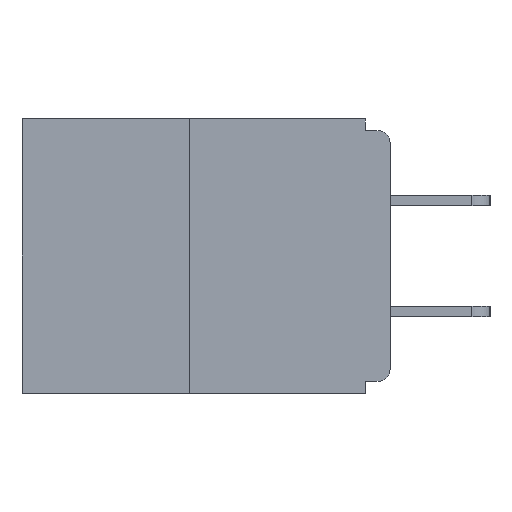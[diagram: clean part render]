
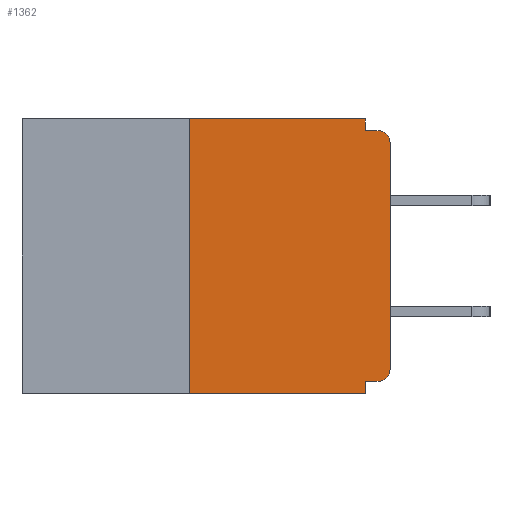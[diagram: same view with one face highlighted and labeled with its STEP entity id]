
A CAD part, left-side view. The second image highlights one B-rep face of the part: STEP entity #1362.
In plain terms, the highlighted planar face has unit normal (-1, 0, 0).
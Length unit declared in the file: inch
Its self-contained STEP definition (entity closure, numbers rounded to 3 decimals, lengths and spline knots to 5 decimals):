
#158 = LINE ( 'NONE', #11465, #11096 ) ;
#204 = DIRECTION ( 'NONE',  ( -1., 0., 0. ) ) ;
#571 = ORIENTED_EDGE ( 'NONE', *, *, #6192, .F. ) ;
#723 = AXIS2_PLACEMENT_3D ( 'NONE', #12080, #2007, #2916 ) ;
#763 = PLANE ( 'NONE',  #6001 ) ;
#1172 = LINE ( 'NONE', #11115, #5064 ) ;
#1209 = CARTESIAN_POINT ( 'NONE',  ( 0., 0.015, -0.313 ) ) ;
#1335 = CARTESIAN_POINT ( 'NONE',  ( 0., 0.25, 0. ) ) ;
#1362 = ADVANCED_FACE ( 'NONE', ( #8601 ), #763, .F. ) ;
#1392 = LINE ( 'NONE', #1335, #8775 ) ;
#1396 = EDGE_CURVE ( 'NONE', #1582, #2213, #1859, .T. ) ;
#1582 = VERTEX_POINT ( 'NONE', #6487 ) ;
#1833 = CARTESIAN_POINT ( 'NONE',  ( 0., 0., 0. ) ) ;
#1859 = LINE ( 'NONE', #5750, #3708 ) ;
#1931 = VECTOR ( 'NONE', #9138, 39.37008 ) ;
#1960 = LINE ( 'NONE', #12014, #11684 ) ;
#2007 = DIRECTION ( 'NONE',  ( -1., 0., 0. ) ) ;
#2177 = DIRECTION ( 'NONE',  ( 0., -1., 0. ) ) ;
#2213 = VERTEX_POINT ( 'NONE', #9863 ) ;
#2240 = VERTEX_POINT ( 'NONE', #11836 ) ;
#2329 = ORIENTED_EDGE ( 'NONE', *, *, #9199, .F. ) ;
#2422 = EDGE_CURVE ( 'NONE', #8087, #2213, #12894, .T. ) ;
#2466 = ORIENTED_EDGE ( 'NONE', *, *, #7427, .F. ) ;
#2494 = VERTEX_POINT ( 'NONE', #4158 ) ;
#2528 = CARTESIAN_POINT ( 'NONE',  ( 0., 0.015, -0.328 ) ) ;
#2592 = ORIENTED_EDGE ( 'NONE', *, *, #1396, .T. ) ;
#2661 = VERTEX_POINT ( 'NONE', #2528 ) ;
#2715 = CIRCLE ( 'NONE', #6135, 0.015 ) ;
#2916 = DIRECTION ( 'NONE',  ( 0., 0., -1. ) ) ;
#3467 = VERTEX_POINT ( 'NONE', #4753 ) ;
#3644 = ORIENTED_EDGE ( 'NONE', *, *, #7300, .T. ) ;
#3673 = DIRECTION ( 'NONE',  ( 0., 0., -1. ) ) ;
#3708 = VECTOR ( 'NONE', #7577, 39.37008 ) ;
#3961 = EDGE_LOOP ( 'NONE', ( #2466, #2329, #2592, #5324, #8359, #8198, #5655, #3644, #4565, #571 ) ) ;
#4158 = CARTESIAN_POINT ( 'NONE',  ( 0., 0., -0.03 ) ) ;
#4565 = ORIENTED_EDGE ( 'NONE', *, *, #8077, .F. ) ;
#4753 = CARTESIAN_POINT ( 'NONE',  ( 0., 0., -0.313 ) ) ;
#4795 = DIRECTION ( 'NONE',  ( 0., 1., 0. ) ) ;
#4956 = DIRECTION ( 'NONE',  ( 0., 0., 1. ) ) ;
#5064 = VECTOR ( 'NONE', #2177, 39.37008 ) ;
#5247 = CARTESIAN_POINT ( 'NONE',  ( 0., 0.031, -0.343 ) ) ;
#5324 = ORIENTED_EDGE ( 'NONE', *, *, #2422, .F. ) ;
#5332 = DIRECTION ( 'NONE',  ( 0., 0., -1. ) ) ;
#5392 = LINE ( 'NONE', #12874, #10449 ) ;
#5416 = DIRECTION ( 'NONE',  ( 0., 0., 1. ) ) ;
#5655 = ORIENTED_EDGE ( 'NONE', *, *, #8929, .T. ) ;
#5750 = CARTESIAN_POINT ( 'NONE',  ( 0., 0.46, -0.343 ) ) ;
#6001 = AXIS2_PLACEMENT_3D ( 'NONE', #11673, #10699, #3673 ) ;
#6135 = AXIS2_PLACEMENT_3D ( 'NONE', #1209, #204, #9180 ) ;
#6192 = EDGE_CURVE ( 'NONE', #2240, #10383, #158, .T. ) ;
#6487 = CARTESIAN_POINT ( 'NONE',  ( 0., 0.25, -0.343 ) ) ;
#6508 = CARTESIAN_POINT ( 'NONE',  ( 0., 0.015, -0.015 ) ) ;
#7300 = EDGE_CURVE ( 'NONE', #2494, #10951, #9175, .T. ) ;
#7427 = EDGE_CURVE ( 'NONE', #9591, #2240, #1172, .T. ) ;
#7447 = CARTESIAN_POINT ( 'NONE',  ( 0., 0.031, -0.015 ) ) ;
#7577 = DIRECTION ( 'NONE',  ( 0., -1., 0. ) ) ;
#8077 = EDGE_CURVE ( 'NONE', #10383, #10951, #1960, .T. ) ;
#8087 = VERTEX_POINT ( 'NONE', #10831 ) ;
#8198 = ORIENTED_EDGE ( 'NONE', *, *, #8713, .T. ) ;
#8247 = CARTESIAN_POINT ( 'NONE',  ( 0., 0.25, 0. ) ) ;
#8359 = ORIENTED_EDGE ( 'NONE', *, *, #11130, .F. ) ;
#8601 = FACE_OUTER_BOUND ( 'NONE', #3961, .T. ) ;
#8713 = EDGE_CURVE ( 'NONE', #2661, #3467, #2715, .T. ) ;
#8775 = VECTOR ( 'NONE', #5416, 39.37008 ) ;
#8929 = EDGE_CURVE ( 'NONE', #3467, #2494, #11355, .T. ) ;
#8990 = DIRECTION ( 'NONE',  ( 0., -1., 0. ) ) ;
#9138 = DIRECTION ( 'NONE',  ( 0., 0., -1. ) ) ;
#9175 = CIRCLE ( 'NONE', #723, 0.015 ) ;
#9180 = DIRECTION ( 'NONE',  ( 0., 0., -1. ) ) ;
#9199 = EDGE_CURVE ( 'NONE', #1582, #9591, #1392, .T. ) ;
#9538 = VECTOR ( 'NONE', #4956, 39.37008 ) ;
#9591 = VERTEX_POINT ( 'NONE', #8247 ) ;
#9863 = CARTESIAN_POINT ( 'NONE',  ( 0., 0.031, -0.343 ) ) ;
#10383 = VERTEX_POINT ( 'NONE', #7447 ) ;
#10449 = VECTOR ( 'NONE', #4795, 39.37008 ) ;
#10699 = DIRECTION ( 'NONE',  ( 1., 0., 0. ) ) ;
#10831 = CARTESIAN_POINT ( 'NONE',  ( 0., 0.031, -0.328 ) ) ;
#10951 = VERTEX_POINT ( 'NONE', #6508 ) ;
#11096 = VECTOR ( 'NONE', #5332, 39.37008 ) ;
#11115 = CARTESIAN_POINT ( 'NONE',  ( 0., 0.46, 0. ) ) ;
#11130 = EDGE_CURVE ( 'NONE', #2661, #8087, #5392, .T. ) ;
#11355 = LINE ( 'NONE', #1833, #9538 ) ;
#11465 = CARTESIAN_POINT ( 'NONE',  ( 0., 0.031, 0. ) ) ;
#11673 = CARTESIAN_POINT ( 'NONE',  ( 0., 0.46, 0. ) ) ;
#11684 = VECTOR ( 'NONE', #8990, 39.37008 ) ;
#11836 = CARTESIAN_POINT ( 'NONE',  ( 0., 0.031, 0. ) ) ;
#12014 = CARTESIAN_POINT ( 'NONE',  ( 0., 0., -0.015 ) ) ;
#12080 = CARTESIAN_POINT ( 'NONE',  ( 0., 0.015, -0.03 ) ) ;
#12874 = CARTESIAN_POINT ( 'NONE',  ( 0., 0., -0.328 ) ) ;
#12894 = LINE ( 'NONE', #5247, #1931 ) ;
